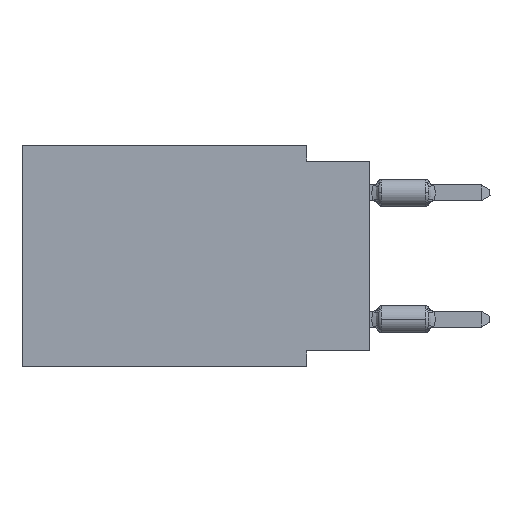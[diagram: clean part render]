
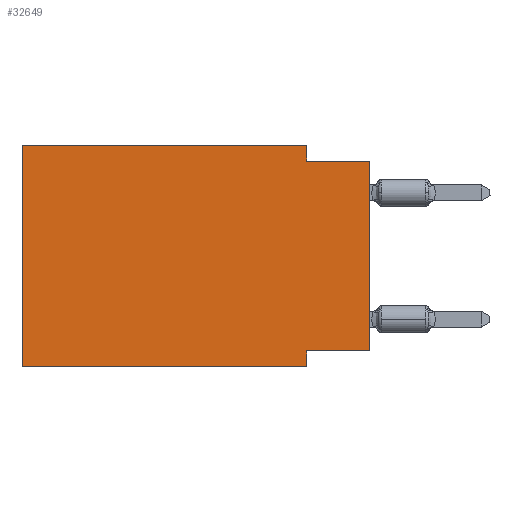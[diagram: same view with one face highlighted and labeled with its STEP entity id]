
A CAD part, left-side view. The second image highlights one B-rep face of the part: STEP entity #32649.
In plain terms, the highlighted planar face has unit normal (-1, 0, 0).
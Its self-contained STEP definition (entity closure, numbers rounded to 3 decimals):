
#696 = VERTEX_POINT ( 'NONE', #6036 ) ;
#1266 = CARTESIAN_POINT ( 'NONE',  ( 0., 13.97, 0. ) ) ;
#1622 = VERTEX_POINT ( 'NONE', #43125 ) ;
#2484 = VECTOR ( 'NONE', #51764, 1000. ) ;
#3534 = CARTESIAN_POINT ( 'NONE',  ( 0., 0., -8.255 ) ) ;
#3893 = LINE ( 'NONE', #44070, #47005 ) ;
#4332 = ORIENTED_EDGE ( 'NONE', *, *, #13141, .T. ) ;
#4359 = VERTEX_POINT ( 'NONE', #13024 ) ;
#5356 = AXIS2_PLACEMENT_3D ( 'NONE', #1266, #17953, #40042 ) ;
#5695 = VERTEX_POINT ( 'NONE', #35614 ) ;
#6036 = CARTESIAN_POINT ( 'NONE',  ( 0., 13.97, -8.89 ) ) ;
#7638 = CARTESIAN_POINT ( 'NONE',  ( 0., 13.97, -8.89 ) ) ;
#11886 = VECTOR ( 'NONE', #32435, 1000. ) ;
#12786 = DIRECTION ( 'NONE',  ( 0., -1., 0. ) ) ;
#13024 = CARTESIAN_POINT ( 'NONE',  ( 0., 2.54, -8.255 ) ) ;
#13141 = EDGE_CURVE ( 'NONE', #52517, #1622, #39386, .T. ) ;
#13522 = ORIENTED_EDGE ( 'NONE', *, *, #46839, .F. ) ;
#14036 = VECTOR ( 'NONE', #15064, 1000. ) ;
#14916 = CARTESIAN_POINT ( 'NONE',  ( 0., 0., -0.635 ) ) ;
#15064 = DIRECTION ( 'NONE',  ( 0., 0., -1. ) ) ;
#15413 = EDGE_CURVE ( 'NONE', #696, #5695, #52119, .T. ) ;
#17125 = DIRECTION ( 'NONE',  ( 0., 0., -1. ) ) ;
#17953 = DIRECTION ( 'NONE',  ( 1., 0., 0. ) ) ;
#18253 = ORIENTED_EDGE ( 'NONE', *, *, #15413, .T. ) ;
#19240 = CARTESIAN_POINT ( 'NONE',  ( 0., 0., -8.255 ) ) ;
#21886 = CARTESIAN_POINT ( 'NONE',  ( 0., 0., 0. ) ) ;
#26646 = VECTOR ( 'NONE', #43694, 1000. ) ;
#26666 = ORIENTED_EDGE ( 'NONE', *, *, #54837, .F. ) ;
#26827 = ORIENTED_EDGE ( 'NONE', *, *, #46851, .F. ) ;
#27130 = FACE_OUTER_BOUND ( 'NONE', #32104, .T. ) ;
#27146 = EDGE_CURVE ( 'NONE', #4359, #5695, #3893, .T. ) ;
#28190 = CARTESIAN_POINT ( 'NONE',  ( 0., 13.97, 0. ) ) ;
#28536 = VERTEX_POINT ( 'NONE', #51723 ) ;
#30231 = LINE ( 'NONE', #3534, #2484 ) ;
#31206 = CARTESIAN_POINT ( 'NONE',  ( 0., 2.54, 0. ) ) ;
#32104 = EDGE_LOOP ( 'NONE', ( #4332, #49220, #26827, #13522, #33053, #18253, #43716, #26666 ) ) ;
#32435 = DIRECTION ( 'NONE',  ( 0., -1., 0. ) ) ;
#32649 = ADVANCED_FACE ( 'NONE', ( #27130 ), #39472, .F. ) ;
#33053 = ORIENTED_EDGE ( 'NONE', *, *, #55152, .F. ) ;
#33625 = EDGE_CURVE ( 'NONE', #28536, #1622, #41608, .T. ) ;
#35614 = CARTESIAN_POINT ( 'NONE',  ( 0., 2.54, -8.89 ) ) ;
#39386 = LINE ( 'NONE', #21886, #26646 ) ;
#39472 = PLANE ( 'NONE',  #5356 ) ;
#39863 = CARTESIAN_POINT ( 'NONE',  ( 0., 13.97, 0. ) ) ;
#40042 = DIRECTION ( 'NONE',  ( 0., 0., -1. ) ) ;
#40356 = VERTEX_POINT ( 'NONE', #39863 ) ;
#41461 = CARTESIAN_POINT ( 'NONE',  ( 0., 2.54, 0. ) ) ;
#41608 = LINE ( 'NONE', #14916, #11886 ) ;
#41944 = DIRECTION ( 'NONE',  ( 0., 0., 1. ) ) ;
#42028 = LINE ( 'NONE', #46341, #55290 ) ;
#43125 = CARTESIAN_POINT ( 'NONE',  ( 0., 0., -0.635 ) ) ;
#43694 = DIRECTION ( 'NONE',  ( 0., 0., 1. ) ) ;
#43716 = ORIENTED_EDGE ( 'NONE', *, *, #27146, .F. ) ;
#44070 = CARTESIAN_POINT ( 'NONE',  ( 0., 2.54, -8.89 ) ) ;
#44123 = VERTEX_POINT ( 'NONE', #31206 ) ;
#44357 = VECTOR ( 'NONE', #12786, 1000. ) ;
#45099 = LINE ( 'NONE', #28190, #48228 ) ;
#46341 = CARTESIAN_POINT ( 'NONE',  ( 0., 13.97, 0. ) ) ;
#46839 = EDGE_CURVE ( 'NONE', #40356, #44123, #42028, .T. ) ;
#46851 = EDGE_CURVE ( 'NONE', #44123, #28536, #50638, .T. ) ;
#47005 = VECTOR ( 'NONE', #17125, 1000. ) ;
#48228 = VECTOR ( 'NONE', #41944, 1000. ) ;
#49220 = ORIENTED_EDGE ( 'NONE', *, *, #33625, .F. ) ;
#49800 = DIRECTION ( 'NONE',  ( 0., -1., 0. ) ) ;
#50638 = LINE ( 'NONE', #41461, #14036 ) ;
#51723 = CARTESIAN_POINT ( 'NONE',  ( 0., 2.54, -0.635 ) ) ;
#51764 = DIRECTION ( 'NONE',  ( 0., 1., 0. ) ) ;
#52119 = LINE ( 'NONE', #7638, #44357 ) ;
#52517 = VERTEX_POINT ( 'NONE', #19240 ) ;
#54837 = EDGE_CURVE ( 'NONE', #52517, #4359, #30231, .T. ) ;
#55152 = EDGE_CURVE ( 'NONE', #696, #40356, #45099, .T. ) ;
#55290 = VECTOR ( 'NONE', #49800, 1000. ) ;
